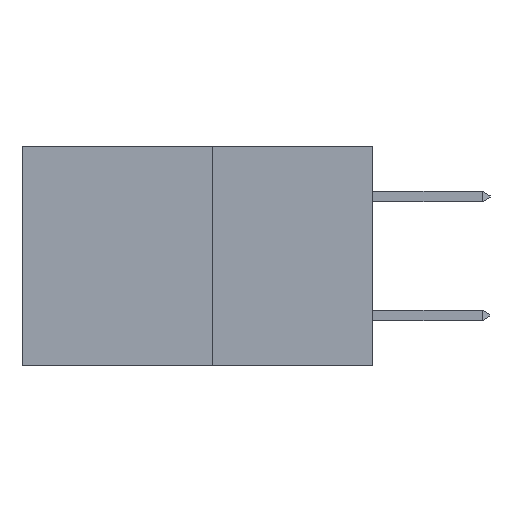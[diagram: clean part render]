
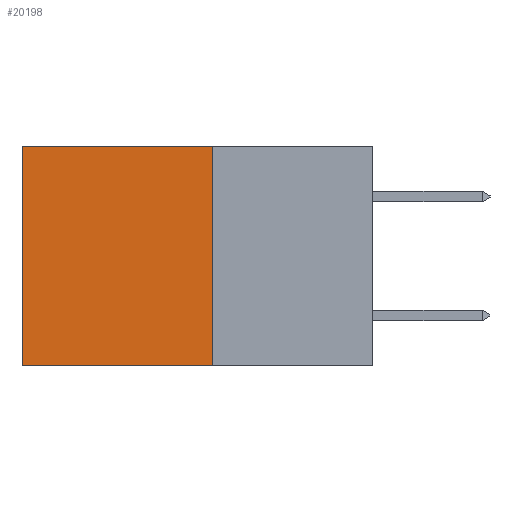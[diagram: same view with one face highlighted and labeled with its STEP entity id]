
A CAD part, left-side view. The second image highlights one B-rep face of the part: STEP entity #20198.
In plain terms, the highlighted planar face has unit normal (-1, 0, 0).
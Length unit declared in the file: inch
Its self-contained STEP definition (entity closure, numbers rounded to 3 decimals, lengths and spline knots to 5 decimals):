
#357 = VERTEX_POINT ( 'NONE', #21323 ) ;
#584 = ORIENTED_EDGE ( 'NONE', *, *, #10136, .T. ) ;
#1232 = AXIS2_PLACEMENT_3D ( 'NONE', #1676, #14939, #3586 ) ;
#1281 = CARTESIAN_POINT ( 'NONE',  ( 0.277, 0.27, -0.37 ) ) ;
#1676 = CARTESIAN_POINT ( 'NONE',  ( 0.277, 0.27, -0.37 ) ) ;
#2070 = VECTOR ( 'NONE', #19695, 39.37008 ) ;
#3196 = DIRECTION ( 'NONE',  ( 0., 0., -1. ) ) ;
#3586 = DIRECTION ( 'NONE',  ( 0., 0., -1. ) ) ;
#5641 = EDGE_CURVE ( 'NONE', #10163, #20752, #15273, .T. ) ;
#6165 = VECTOR ( 'NONE', #10637, 39.37008 ) ;
#6427 = VECTOR ( 'NONE', #3196, 39.37008 ) ;
#6540 = LINE ( 'NONE', #23520, #2070 ) ;
#6753 = LINE ( 'NONE', #8709, #6165 ) ;
#7418 = ORIENTED_EDGE ( 'NONE', *, *, #14537, .F. ) ;
#8362 = ORIENTED_EDGE ( 'NONE', *, *, #5641, .F. ) ;
#8709 = CARTESIAN_POINT ( 'NONE',  ( 0.277, 0.59, -0.37 ) ) ;
#10136 = EDGE_CURVE ( 'NONE', #23992, #357, #6540, .T. ) ;
#10163 = VERTEX_POINT ( 'NONE', #12113 ) ;
#10637 = DIRECTION ( 'NONE',  ( 0., 0., -1. ) ) ;
#10960 = DIRECTION ( 'NONE',  ( 0., 1., 0. ) ) ;
#11893 = FACE_OUTER_BOUND ( 'NONE', #17838, .T. ) ;
#12113 = CARTESIAN_POINT ( 'NONE',  ( 0.277, 0.27, -0.37 ) ) ;
#13034 = PLANE ( 'NONE',  #1232 ) ;
#14429 = CARTESIAN_POINT ( 'NONE',  ( 0.277, 0.27, 0. ) ) ;
#14537 = EDGE_CURVE ( 'NONE', #23992, #10163, #17730, .T. ) ;
#14939 = DIRECTION ( 'NONE',  ( 1., 0., 0. ) ) ;
#15273 = LINE ( 'NONE', #20465, #19779 ) ;
#16411 = CARTESIAN_POINT ( 'NONE',  ( 0.277, 0.59, -0.37 ) ) ;
#17730 = LINE ( 'NONE', #1281, #6427 ) ;
#17838 = EDGE_LOOP ( 'NONE', ( #23599, #8362, #7418, #584 ) ) ;
#19695 = DIRECTION ( 'NONE',  ( 0., 1., 0. ) ) ;
#19779 = VECTOR ( 'NONE', #10960, 39.37008 ) ;
#20198 = ADVANCED_FACE ( 'NONE', ( #11893 ), #13034, .F. ) ;
#20465 = CARTESIAN_POINT ( 'NONE',  ( 0.277, 0.27, -0.37 ) ) ;
#20752 = VERTEX_POINT ( 'NONE', #16411 ) ;
#21323 = CARTESIAN_POINT ( 'NONE',  ( 0.277, 0.59, 0. ) ) ;
#22011 = EDGE_CURVE ( 'NONE', #357, #20752, #6753, .T. ) ;
#23520 = CARTESIAN_POINT ( 'NONE',  ( 0.277, 0.27, 0. ) ) ;
#23599 = ORIENTED_EDGE ( 'NONE', *, *, #22011, .T. ) ;
#23992 = VERTEX_POINT ( 'NONE', #14429 ) ;
